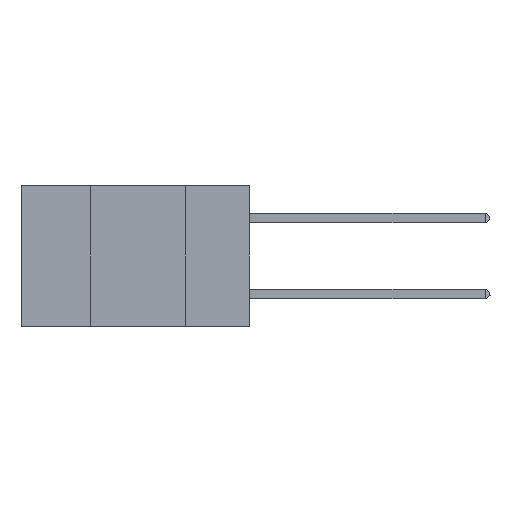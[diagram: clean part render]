
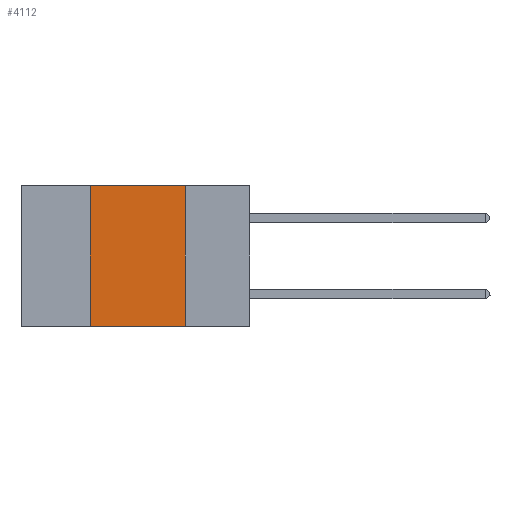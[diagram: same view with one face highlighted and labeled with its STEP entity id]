
A CAD part, left-side view. The second image highlights one B-rep face of the part: STEP entity #4112.
In plain terms, the highlighted planar face has unit normal (-1, 0, 0).
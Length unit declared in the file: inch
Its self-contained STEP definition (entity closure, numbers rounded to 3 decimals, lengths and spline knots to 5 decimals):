
#77 = VECTOR ( 'NONE', #5396, 39.37008 ) ;
#83 = ORIENTED_EDGE ( 'NONE', *, *, #11736, .T. ) ;
#561 = LINE ( 'NONE', #16706, #4501 ) ;
#865 = ORIENTED_EDGE ( 'NONE', *, *, #17816, .F. ) ;
#1246 = CARTESIAN_POINT ( 'NONE',  ( 0., 0.17, 0. ) ) ;
#1898 = LINE ( 'NONE', #7737, #3213 ) ;
#2979 = VERTEX_POINT ( 'NONE', #15702 ) ;
#3213 = VECTOR ( 'NONE', #14549, 39.37008 ) ;
#3273 = VECTOR ( 'NONE', #13638, 39.37008 ) ;
#3274 = EDGE_CURVE ( 'NONE', #14132, #11404, #7296, .T. ) ;
#3572 = PLANE ( 'NONE',  #15744 ) ;
#3702 = ORIENTED_EDGE ( 'NONE', *, *, #3274, .F. ) ;
#3974 = DIRECTION ( 'NONE',  ( 0., 0., 1. ) ) ;
#4112 = ADVANCED_FACE ( 'NONE', ( #9943 ), #3572, .F. ) ;
#4501 = VECTOR ( 'NONE', #3974, 39.37008 ) ;
#5396 = DIRECTION ( 'NONE',  ( 0., 0., -1. ) ) ;
#6326 = VERTEX_POINT ( 'NONE', #6708 ) ;
#6708 = CARTESIAN_POINT ( 'NONE',  ( 0., 0.42, -0.37 ) ) ;
#7174 = EDGE_CURVE ( 'NONE', #2979, #14132, #1898, .T. ) ;
#7296 = LINE ( 'NONE', #1246, #77 ) ;
#7737 = CARTESIAN_POINT ( 'NONE',  ( 0., 0.6, 0. ) ) ;
#9092 = CARTESIAN_POINT ( 'NONE',  ( 0., 0.6, 0. ) ) ;
#9943 = FACE_OUTER_BOUND ( 'NONE', #10629, .T. ) ;
#10629 = EDGE_LOOP ( 'NONE', ( #3702, #15608, #865, #83 ) ) ;
#11404 = VERTEX_POINT ( 'NONE', #12550 ) ;
#11736 = EDGE_CURVE ( 'NONE', #6326, #11404, #13800, .T. ) ;
#12550 = CARTESIAN_POINT ( 'NONE',  ( 0., 0.17, -0.37 ) ) ;
#13356 = DIRECTION ( 'NONE',  ( 1., 0., 0. ) ) ;
#13638 = DIRECTION ( 'NONE',  ( 0., -1., 0. ) ) ;
#13800 = LINE ( 'NONE', #17834, #3273 ) ;
#14132 = VERTEX_POINT ( 'NONE', #16002 ) ;
#14549 = DIRECTION ( 'NONE',  ( 0., -1., 0. ) ) ;
#14775 = DIRECTION ( 'NONE',  ( 0., 0., -1. ) ) ;
#15608 = ORIENTED_EDGE ( 'NONE', *, *, #7174, .F. ) ;
#15702 = CARTESIAN_POINT ( 'NONE',  ( 0., 0.42, 0. ) ) ;
#15744 = AXIS2_PLACEMENT_3D ( 'NONE', #9092, #13356, #14775 ) ;
#16002 = CARTESIAN_POINT ( 'NONE',  ( 0., 0.17, 0. ) ) ;
#16706 = CARTESIAN_POINT ( 'NONE',  ( 0., 0.42, 0. ) ) ;
#17816 = EDGE_CURVE ( 'NONE', #6326, #2979, #561, .T. ) ;
#17834 = CARTESIAN_POINT ( 'NONE',  ( 0., 0.6, -0.37 ) ) ;
